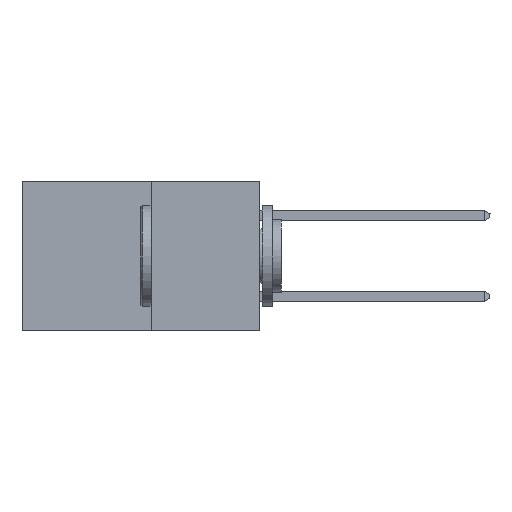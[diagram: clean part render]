
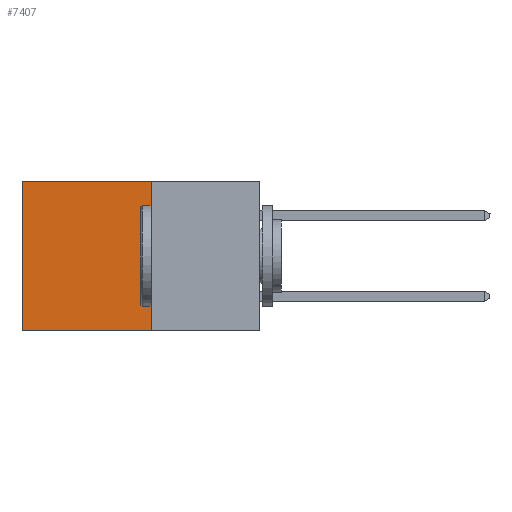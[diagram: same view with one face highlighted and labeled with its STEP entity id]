
A CAD part, left-side view. The second image highlights one B-rep face of the part: STEP entity #7407.
In plain terms, the highlighted planar face has unit normal (-1, 0, 0).
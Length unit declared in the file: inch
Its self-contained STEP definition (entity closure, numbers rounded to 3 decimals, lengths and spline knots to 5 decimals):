
#15 = VERTEX_POINT ( 'NONE', #8812 ) ;
#550 = DIRECTION ( 'NONE',  ( 0., 1., 0. ) ) ;
#613 = CARTESIAN_POINT ( 'NONE',  ( 0.277, 0.27, 0. ) ) ;
#1170 = LINE ( 'NONE', #5439, #3267 ) ;
#1250 = VECTOR ( 'NONE', #550, 39.37008 ) ;
#1604 = CARTESIAN_POINT ( 'NONE',  ( 0.277, 0.27, -0.37 ) ) ;
#1963 = VERTEX_POINT ( 'NONE', #10263 ) ;
#3027 = DIRECTION ( 'NONE',  ( 0., 0., -1. ) ) ;
#3259 = CARTESIAN_POINT ( 'NONE',  ( 0.277, 0.59, -0.37 ) ) ;
#3267 = VECTOR ( 'NONE', #5545, 39.37008 ) ;
#4089 = EDGE_LOOP ( 'NONE', ( #8766, #11364, #6217, #11124 ) ) ;
#4096 = AXIS2_PLACEMENT_3D ( 'NONE', #10756, #10321, #10311 ) ;
#4352 = VERTEX_POINT ( 'NONE', #9941 ) ;
#5065 = EDGE_CURVE ( 'NONE', #6092, #15, #8896, .T. ) ;
#5235 = LINE ( 'NONE', #3259, #9792 ) ;
#5439 = CARTESIAN_POINT ( 'NONE',  ( 0.277, 0.27, -0.37 ) ) ;
#5545 = DIRECTION ( 'NONE',  ( 0., 0., -1. ) ) ;
#6092 = VERTEX_POINT ( 'NONE', #1604 ) ;
#6217 = ORIENTED_EDGE ( 'NONE', *, *, #8514, .F. ) ;
#7141 = EDGE_CURVE ( 'NONE', #4352, #15, #5235, .T. ) ;
#7407 = ADVANCED_FACE ( 'NONE', ( #8102 ), #10377, .F. ) ;
#8102 = FACE_OUTER_BOUND ( 'NONE', #4089, .T. ) ;
#8514 = EDGE_CURVE ( 'NONE', #1963, #6092, #1170, .T. ) ;
#8766 = ORIENTED_EDGE ( 'NONE', *, *, #7141, .T. ) ;
#8812 = CARTESIAN_POINT ( 'NONE',  ( 0.277, 0.59, -0.37 ) ) ;
#8896 = LINE ( 'NONE', #9768, #11219 ) ;
#9768 = CARTESIAN_POINT ( 'NONE',  ( 0.277, 0.27, -0.37 ) ) ;
#9792 = VECTOR ( 'NONE', #3027, 39.37008 ) ;
#9941 = CARTESIAN_POINT ( 'NONE',  ( 0.277, 0.59, 0. ) ) ;
#10237 = DIRECTION ( 'NONE',  ( 0., 1., 0. ) ) ;
#10258 = LINE ( 'NONE', #613, #1250 ) ;
#10263 = CARTESIAN_POINT ( 'NONE',  ( 0.277, 0.27, 0. ) ) ;
#10311 = DIRECTION ( 'NONE',  ( 0., 0., -1. ) ) ;
#10321 = DIRECTION ( 'NONE',  ( 1., 0., 0. ) ) ;
#10377 = PLANE ( 'NONE',  #4096 ) ;
#10756 = CARTESIAN_POINT ( 'NONE',  ( 0.277, 0.27, -0.37 ) ) ;
#11003 = EDGE_CURVE ( 'NONE', #1963, #4352, #10258, .T. ) ;
#11124 = ORIENTED_EDGE ( 'NONE', *, *, #11003, .T. ) ;
#11219 = VECTOR ( 'NONE', #10237, 39.37008 ) ;
#11364 = ORIENTED_EDGE ( 'NONE', *, *, #5065, .F. ) ;
